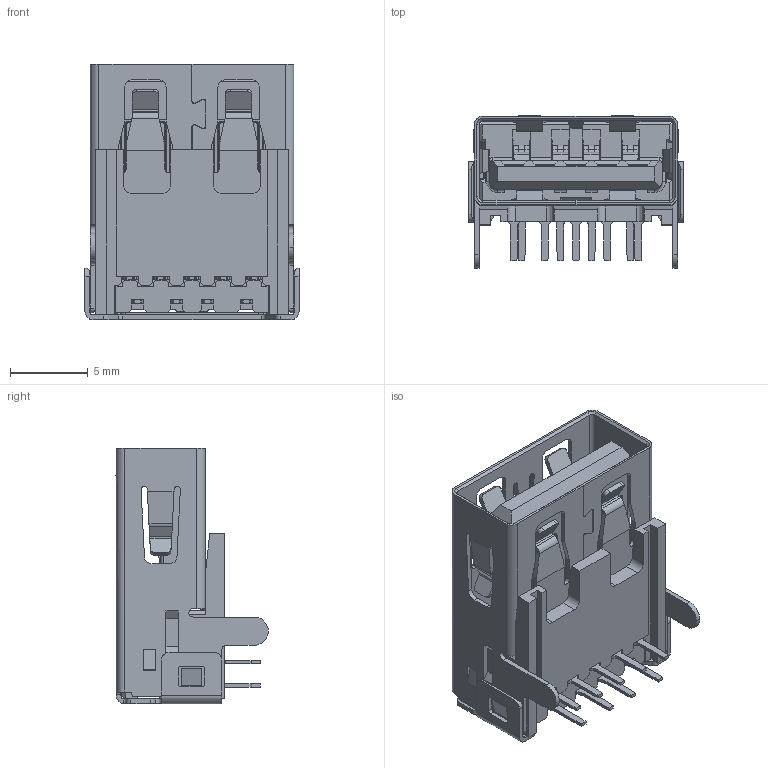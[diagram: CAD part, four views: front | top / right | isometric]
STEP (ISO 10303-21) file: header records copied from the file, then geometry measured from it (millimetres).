
FILE_DESCRIPTION (( 'STEP AP214' ), '1' );
FILE_NAME ('690B509-221-226.STEP', '2021-01-14T17:45:07', ( '' ), ( '' ), 'SwSTEP 2.0', 'SolidWorks 2020', '' );
FILE_SCHEMA (( 'AUTOMOTIVE_DESIGN' ));
Length unit declared in the file: millimetre
Products named in the file (8): Insulator2 690B509-221-226; Contact 2.0 4 690B509-221-226; Contact 2.0 1 690B509-221-226; Contact 2.0 690B509-221-226; 690B509-221-226; Insulator1 690B509-221-226; Contact 3.0 690B509-221-226; Shell 690B509-221-226
Assembly tree (12 placements, depth 2):
  690B509-221-226
    Insulator1 690B509-221-226
    Contact 3.0 690B509-221-226  x5
    Insulator2 690B509-221-226
    Shell 690B509-221-226
    Contact 2.0 1 690B509-221-226
    Contact 2.0 690B509-221-226  x2
    Contact 2.0 4 690B509-221-226
Bounding box: 13.8 x 9.83 x 16.45 mm (x, y, z)
Volume: 666.4 mm3; surface area: 3051.8 mm2
Topology: 12 solids, 12 shells, 2409 faces, 6913 edges, 4509 vertices
Faces by surface type: plane 1582, cylinder 705, bspline 118, cone 4
Entity records: 61118 total; most frequent: CARTESIAN_POINT 12724, ORIENTED_EDGE 10534, DIRECTION 9480, EDGE_CURVE 5267, LINE 4182, VECTOR 4182, VERTEX_POINT 3435, AXIS2_PLACEMENT_3D 2649
